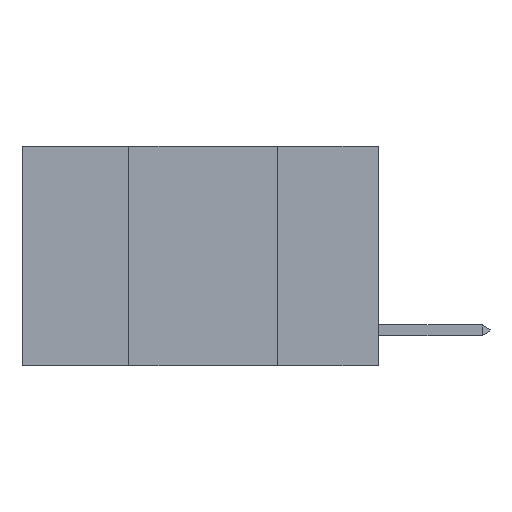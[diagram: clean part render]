
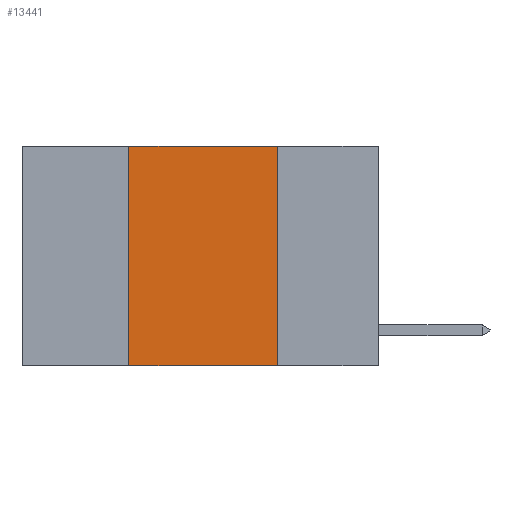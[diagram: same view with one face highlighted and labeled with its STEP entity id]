
A CAD part, left-side view. The second image highlights one B-rep face of the part: STEP entity #13441.
In plain terms, the highlighted planar face has unit normal (-1, 0, 0).
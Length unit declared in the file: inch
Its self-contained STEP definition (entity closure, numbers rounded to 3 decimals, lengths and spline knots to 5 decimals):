
#21 = VERTEX_POINT ( 'NONE', #14404 ) ;
#642 = CARTESIAN_POINT ( 'NONE',  ( 0., 0.6, -0.37 ) ) ;
#2669 = DIRECTION ( 'NONE',  ( 0., -1., 0. ) ) ;
#3485 = VECTOR ( 'NONE', #13231, 39.37008 ) ;
#3912 = ORIENTED_EDGE ( 'NONE', *, *, #27017, .F. ) ;
#4896 = ORIENTED_EDGE ( 'NONE', *, *, #21162, .F. ) ;
#5479 = LINE ( 'NONE', #642, #3485 ) ;
#8735 = PLANE ( 'NONE',  #11331 ) ;
#9084 = CARTESIAN_POINT ( 'NONE',  ( 0., 0.17, 0. ) ) ;
#10863 = DIRECTION ( 'NONE',  ( 1., 0., 0. ) ) ;
#11331 = AXIS2_PLACEMENT_3D ( 'NONE', #21363, #10863, #25621 ) ;
#11985 = VECTOR ( 'NONE', #25954, 39.37008 ) ;
#12195 = ORIENTED_EDGE ( 'NONE', *, *, #15485, .T. ) ;
#13074 = CARTESIAN_POINT ( 'NONE',  ( 0., 0.6, 0. ) ) ;
#13231 = DIRECTION ( 'NONE',  ( 0., -1., 0. ) ) ;
#13441 = ADVANCED_FACE ( 'NONE', ( #15220 ), #8735, .F. ) ;
#14404 = CARTESIAN_POINT ( 'NONE',  ( 0., 0.17, 0. ) ) ;
#15220 = FACE_OUTER_BOUND ( 'NONE', #27039, .T. ) ;
#15485 = EDGE_CURVE ( 'NONE', #18418, #16310, #5479, .T. ) ;
#16310 = VERTEX_POINT ( 'NONE', #20237 ) ;
#16916 = EDGE_CURVE ( 'NONE', #18418, #25152, #22932, .T. ) ;
#17360 = CARTESIAN_POINT ( 'NONE',  ( 0., 0.42, -0.37 ) ) ;
#17565 = LINE ( 'NONE', #9084, #11985 ) ;
#18006 = CARTESIAN_POINT ( 'NONE',  ( 0., 0.42, 0. ) ) ;
#18418 = VERTEX_POINT ( 'NONE', #17360 ) ;
#19140 = DIRECTION ( 'NONE',  ( 0., 0., 1. ) ) ;
#19604 = VECTOR ( 'NONE', #2669, 39.37008 ) ;
#20237 = CARTESIAN_POINT ( 'NONE',  ( 0., 0.17, -0.37 ) ) ;
#20272 = LINE ( 'NONE', #13074, #19604 ) ;
#21162 = EDGE_CURVE ( 'NONE', #21, #16310, #17565, .T. ) ;
#21363 = CARTESIAN_POINT ( 'NONE',  ( 0., 0.6, 0. ) ) ;
#22250 = VECTOR ( 'NONE', #19140, 39.37008 ) ;
#22932 = LINE ( 'NONE', #25028, #22250 ) ;
#23450 = ORIENTED_EDGE ( 'NONE', *, *, #16916, .F. ) ;
#25028 = CARTESIAN_POINT ( 'NONE',  ( 0., 0.42, 0. ) ) ;
#25152 = VERTEX_POINT ( 'NONE', #18006 ) ;
#25621 = DIRECTION ( 'NONE',  ( 0., 0., -1. ) ) ;
#25954 = DIRECTION ( 'NONE',  ( 0., 0., -1. ) ) ;
#27017 = EDGE_CURVE ( 'NONE', #25152, #21, #20272, .T. ) ;
#27039 = EDGE_LOOP ( 'NONE', ( #4896, #3912, #23450, #12195 ) ) ;
